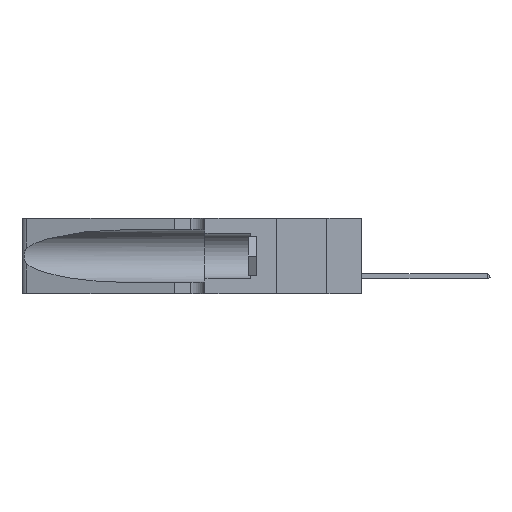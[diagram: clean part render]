
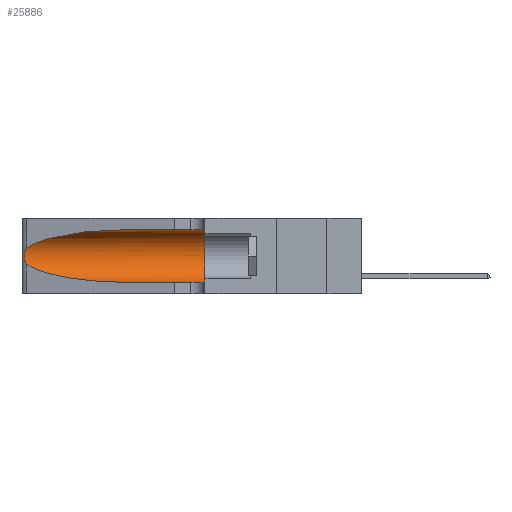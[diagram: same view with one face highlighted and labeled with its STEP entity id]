
A CAD part, left-side view. The second image highlights one B-rep face of the part: STEP entity #25886.
In plain terms, the highlighted cylindrical face has radius 3.308 mm (diameter 6.617 mm), a partial arc.
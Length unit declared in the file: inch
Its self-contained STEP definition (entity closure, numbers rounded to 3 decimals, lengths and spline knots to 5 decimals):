
#168 = CARTESIAN_POINT ( 'NONE',  ( 0.25487, 1.22718, 0.22369 ) ) ;
#199 = CARTESIAN_POINT ( 'NONE',  ( 0.25639, 1.23186, 0.15144 ) ) ;
#484 = VERTEX_POINT ( 'NONE', #2609 ) ;
#1034 = CARTESIAN_POINT ( 'NONE',  ( 0.1305, 1.61858, 0.31525 ) ) ;
#1984 = EDGE_CURVE ( 'NONE', #2347, #4735, #13894, .T. ) ;
#2347 = VERTEX_POINT ( 'NONE', #8930 ) ;
#2609 = CARTESIAN_POINT ( 'NONE',  ( 0.1305, 0.35, 0.05475 ) ) ;
#2849 =( BOUNDED_CURVE ( )  B_SPLINE_CURVE ( 3, ( #23092, #27643, #13689, #168 ),
 .UNSPECIFIED., .F., .T. ) 
 B_SPLINE_CURVE_WITH_KNOTS ( ( 4, 4 ),
 ( 1.5708, 2.84003 ),
 .UNSPECIFIED. ) 
 CURVE ( )  GEOMETRIC_REPRESENTATION_ITEM ( )  RATIONAL_B_SPLINE_CURVE ( ( 1., 0.87, 0.87, 1. ) ) 
 REPRESENTATION_ITEM ( '' )  );
#3002 = FACE_OUTER_BOUND ( 'NONE', #22977, .T. ) ;
#3188 = CARTESIAN_POINT ( 'NONE',  ( 0.1305, 0.72297, 0.05475 ) ) ;
#3441 = EDGE_CURVE ( 'NONE', #5124, #484, #9271, .T. ) ;
#3509 = LINE ( 'NONE', #1034, #21098 ) ;
#4735 = VERTEX_POINT ( 'NONE', #22547 ) ;
#4919 = EDGE_CURVE ( 'NONE', #8878, #484, #23825, .T. ) ;
#5124 = VERTEX_POINT ( 'NONE', #10685 ) ;
#5189 = VECTOR ( 'NONE', #18545, 39.37008 ) ;
#5526 = CYLINDRICAL_SURFACE ( 'NONE', #12021, 0.13025 ) ;
#5585 = CARTESIAN_POINT ( 'NONE',  ( 0.18966, 0.96281, 0.05475 ) ) ;
#6109 = CARTESIAN_POINT ( 'NONE',  ( 0.25787, 1.23484, 0.2124 ) ) ;
#6547 = CARTESIAN_POINT ( 'NONE',  ( 0.1305, 0.72297, 0.31525 ) ) ;
#8316 = CARTESIAN_POINT ( 'NONE',  ( 0.25555, 1.22994, 0.2215 ) ) ;
#8878 = VERTEX_POINT ( 'NONE', #10752 ) ;
#8930 = CARTESIAN_POINT ( 'NONE',  ( 0.25487, 1.22718, 0.22369 ) ) ;
#9271 = CIRCLE ( 'NONE', #12770, 0.13025 ) ;
#9958 = DIRECTION ( 'NONE',  ( 0., 1., 0. ) ) ;
#10432 = CARTESIAN_POINT ( 'NONE',  ( 0.25487, 1.22718, 0.22369 ) ) ;
#10685 = CARTESIAN_POINT ( 'NONE',  ( 0.1305, 0.35, 0.31525 ) ) ;
#10752 = CARTESIAN_POINT ( 'NONE',  ( 0.1305, 0.72297, 0.05475 ) ) ;
#11013 = VERTEX_POINT ( 'NONE', #6547 ) ;
#11209 = CARTESIAN_POINT ( 'NONE',  ( 0.26075, 1.23896, 0.178 ) ) ;
#12021 = AXIS2_PLACEMENT_3D ( 'NONE', #24899, #27359, #25267 ) ;
#12770 = AXIS2_PLACEMENT_3D ( 'NONE', #25925, #9958, #16519 ) ;
#13319 = CARTESIAN_POINT ( 'NONE',  ( 0.26075, 1.23896, 0.19203 ) ) ;
#13689 = CARTESIAN_POINT ( 'NONE',  ( 0.2373, 1.15595, 0.28018 ) ) ;
#13746 = ORIENTED_EDGE ( 'NONE', *, *, #3441, .F. ) ;
#13811 = CARTESIAN_POINT ( 'NONE',  ( 0.25789, 1.23486, 0.15765 ) ) ;
#13894 = B_SPLINE_CURVE_WITH_KNOTS ( 'NONE', 3,
 ( #10432, #8316, #28882, #6109, #26403, #22417, #13319, #11209, #13920, #18437, #13811, #199, #29582, #16243 ),
 .UNSPECIFIED., .F., .F.,
 ( 4, 2, 2, 2, 2, 2, 4 ),
 ( 0., 0.00027, 0.00053, 0.00107, 0.0016, 0.00187, 0.00214 ),
 .UNSPECIFIED. ) ;
#13920 = CARTESIAN_POINT ( 'NONE',  ( 0.26017, 1.23833, 0.17102 ) ) ;
#16243 = CARTESIAN_POINT ( 'NONE',  ( 0.25487, 1.22718, 0.14631 ) ) ;
#16519 = DIRECTION ( 'NONE',  ( 0., 0., 1. ) ) ;
#18411 = EDGE_CURVE ( 'NONE', #11013, #5124, #3509, .T. ) ;
#18433 = ORIENTED_EDGE ( 'NONE', *, *, #4919, .T. ) ;
#18437 = CARTESIAN_POINT ( 'NONE',  ( 0.25856, 1.23593, 0.16098 ) ) ;
#18545 = DIRECTION ( 'NONE',  ( 0., -1., 0. ) ) ;
#19322 = EDGE_CURVE ( 'NONE', #11013, #2347, #2849, .T. ) ;
#19324 = CARTESIAN_POINT ( 'NONE',  ( 0.2373, 1.15595, 0.08982 ) ) ;
#19432 = ORIENTED_EDGE ( 'NONE', *, *, #19322, .T. ) ;
#19550 = EDGE_CURVE ( 'NONE', #4735, #8878, #25926, .T. ) ;
#20345 = ORIENTED_EDGE ( 'NONE', *, *, #18411, .F. ) ;
#20654 = CARTESIAN_POINT ( 'NONE',  ( 0.25487, 1.22718, 0.14631 ) ) ;
#21098 = VECTOR ( 'NONE', #23575, 39.37008 ) ;
#21500 = ORIENTED_EDGE ( 'NONE', *, *, #19550, .T. ) ;
#22417 = CARTESIAN_POINT ( 'NONE',  ( 0.26018, 1.23835, 0.19895 ) ) ;
#22547 = CARTESIAN_POINT ( 'NONE',  ( 0.25487, 1.22718, 0.14631 ) ) ;
#22977 = EDGE_LOOP ( 'NONE', ( #19432, #25213, #21500, #18433, #13746, #20345 ) ) ;
#23092 = CARTESIAN_POINT ( 'NONE',  ( 0.1305, 0.72297, 0.31525 ) ) ;
#23575 = DIRECTION ( 'NONE',  ( 0., -1., 0. ) ) ;
#23825 = LINE ( 'NONE', #25109, #5189 ) ;
#24899 = CARTESIAN_POINT ( 'NONE',  ( 0.1305, 1.61858, 0.185 ) ) ;
#25109 = CARTESIAN_POINT ( 'NONE',  ( 0.1305, 1.61858, 0.05475 ) ) ;
#25213 = ORIENTED_EDGE ( 'NONE', *, *, #1984, .T. ) ;
#25267 = DIRECTION ( 'NONE',  ( 0., 0., -1. ) ) ;
#25886 = ADVANCED_FACE ( 'NONE', ( #3002 ), #5526, .F. ) ;
#25925 = CARTESIAN_POINT ( 'NONE',  ( 0.1305, 0.35, 0.185 ) ) ;
#25926 =( BOUNDED_CURVE ( )  B_SPLINE_CURVE ( 3, ( #20654, #19324, #5585, #3188 ),
 .UNSPECIFIED., .F., .T. ) 
 B_SPLINE_CURVE_WITH_KNOTS ( ( 4, 4 ),
 ( 3.44316, 4.71239 ),
 .UNSPECIFIED. ) 
 CURVE ( )  GEOMETRIC_REPRESENTATION_ITEM ( )  RATIONAL_B_SPLINE_CURVE ( ( 1., 0.87, 0.87, 1. ) ) 
 REPRESENTATION_ITEM ( '' )  );
#26403 = CARTESIAN_POINT ( 'NONE',  ( 0.25854, 1.2359, 0.20912 ) ) ;
#27359 = DIRECTION ( 'NONE',  ( 0., -1., 0. ) ) ;
#27643 = CARTESIAN_POINT ( 'NONE',  ( 0.18966, 0.96281, 0.31525 ) ) ;
#28882 = CARTESIAN_POINT ( 'NONE',  ( 0.25639, 1.23184, 0.21858 ) ) ;
#29582 = CARTESIAN_POINT ( 'NONE',  ( 0.25555, 1.22993, 0.14849 ) ) ;
